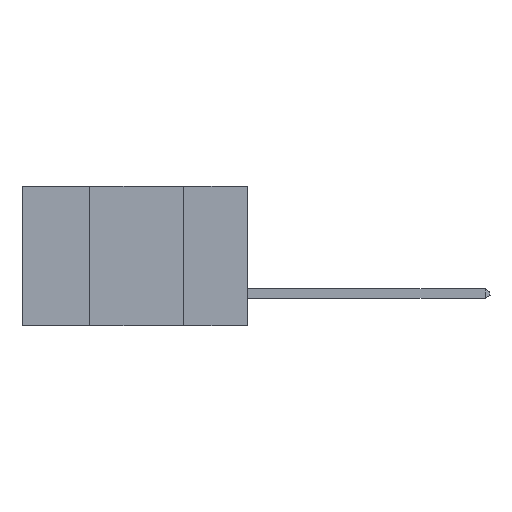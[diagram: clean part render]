
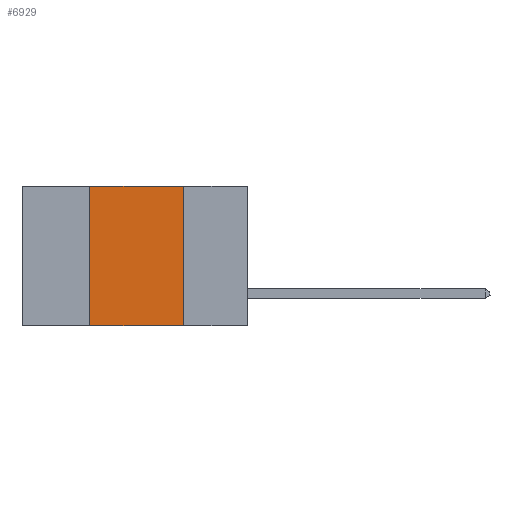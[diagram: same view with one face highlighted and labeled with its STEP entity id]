
A CAD part, left-side view. The second image highlights one B-rep face of the part: STEP entity #6929.
In plain terms, the highlighted planar face has unit normal (-1, 0, 0).
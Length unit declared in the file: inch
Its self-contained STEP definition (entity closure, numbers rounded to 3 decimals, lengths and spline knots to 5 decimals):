
#951 = EDGE_LOOP ( 'NONE', ( #13406, #16619, #14455, #5896 ) ) ;
#1412 = CARTESIAN_POINT ( 'NONE',  ( 0., 0.17, 0. ) ) ;
#1430 = LINE ( 'NONE', #7057, #7310 ) ;
#1556 = CARTESIAN_POINT ( 'NONE',  ( 0., 0.42, -0.37 ) ) ;
#1682 = VECTOR ( 'NONE', #5263, 39.37008 ) ;
#1744 = VERTEX_POINT ( 'NONE', #2510 ) ;
#1779 = EDGE_CURVE ( 'NONE', #2635, #2433, #12605, .T. ) ;
#2194 = LINE ( 'NONE', #19859, #1682 ) ;
#2208 = CARTESIAN_POINT ( 'NONE',  ( 0., 0.6, 0. ) ) ;
#2221 = EDGE_CURVE ( 'NONE', #1744, #14218, #1430, .T. ) ;
#2433 = VERTEX_POINT ( 'NONE', #20557 ) ;
#2510 = CARTESIAN_POINT ( 'NONE',  ( 0., 0.42, 0. ) ) ;
#2635 = VERTEX_POINT ( 'NONE', #1556 ) ;
#2835 = VECTOR ( 'NONE', #10089, 39.37008 ) ;
#4397 = DIRECTION ( 'NONE',  ( 0., 0., -1. ) ) ;
#5203 = AXIS2_PLACEMENT_3D ( 'NONE', #2208, #18872, #4397 ) ;
#5263 = DIRECTION ( 'NONE',  ( 0., 0., 1. ) ) ;
#5701 = CARTESIAN_POINT ( 'NONE',  ( 0., 0.6, -0.37 ) ) ;
#5745 = PLANE ( 'NONE',  #5203 ) ;
#5781 = DIRECTION ( 'NONE',  ( 0., -1., 0. ) ) ;
#5896 = ORIENTED_EDGE ( 'NONE', *, *, #1779, .T. ) ;
#6929 = ADVANCED_FACE ( 'NONE', ( #19538 ), #5745, .F. ) ;
#7057 = CARTESIAN_POINT ( 'NONE',  ( 0., 0.6, 0. ) ) ;
#7191 = LINE ( 'NONE', #18406, #2835 ) ;
#7310 = VECTOR ( 'NONE', #8956, 39.37008 ) ;
#8956 = DIRECTION ( 'NONE',  ( 0., -1., 0. ) ) ;
#10089 = DIRECTION ( 'NONE',  ( 0., 0., -1. ) ) ;
#10090 = EDGE_CURVE ( 'NONE', #2635, #1744, #2194, .T. ) ;
#10598 = VECTOR ( 'NONE', #5781, 39.37008 ) ;
#12605 = LINE ( 'NONE', #5701, #10598 ) ;
#13406 = ORIENTED_EDGE ( 'NONE', *, *, #18771, .F. ) ;
#14218 = VERTEX_POINT ( 'NONE', #1412 ) ;
#14455 = ORIENTED_EDGE ( 'NONE', *, *, #10090, .F. ) ;
#16619 = ORIENTED_EDGE ( 'NONE', *, *, #2221, .F. ) ;
#18406 = CARTESIAN_POINT ( 'NONE',  ( 0., 0.17, 0. ) ) ;
#18771 = EDGE_CURVE ( 'NONE', #14218, #2433, #7191, .T. ) ;
#18872 = DIRECTION ( 'NONE',  ( 1., 0., 0. ) ) ;
#19538 = FACE_OUTER_BOUND ( 'NONE', #951, .T. ) ;
#19859 = CARTESIAN_POINT ( 'NONE',  ( 0., 0.42, 0. ) ) ;
#20557 = CARTESIAN_POINT ( 'NONE',  ( 0., 0.17, -0.37 ) ) ;
